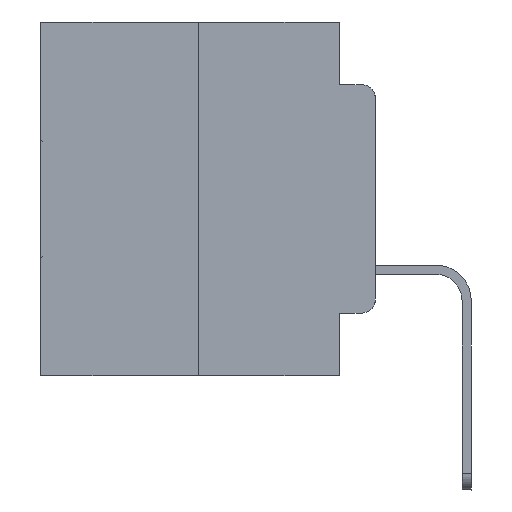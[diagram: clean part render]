
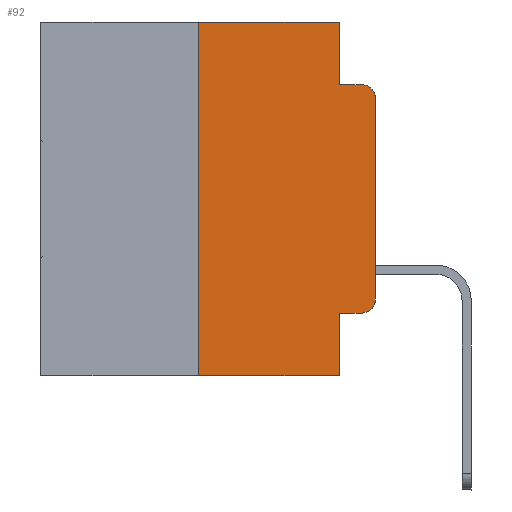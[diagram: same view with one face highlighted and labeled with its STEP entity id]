
A CAD part, left-side view. The second image highlights one B-rep face of the part: STEP entity #92.
In plain terms, the highlighted planar face has unit normal (-1, 0, 0).
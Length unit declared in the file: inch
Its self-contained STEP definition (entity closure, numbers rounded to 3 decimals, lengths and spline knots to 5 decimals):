
#92 = ADVANCED_FACE ( 'NONE', ( #2176 ), #473, .F. ) ;
#256 = EDGE_CURVE ( 'NONE', #11930, #10990, #23237, .T. ) ;
#473 = PLANE ( 'NONE',  #17647 ) ;
#1039 = CARTESIAN_POINT ( 'NONE',  ( 0., 0.051, -0.4115 ) ) ;
#1094 = EDGE_CURVE ( 'NONE', #29498, #14457, #22455, .T. ) ;
#1279 = VERTEX_POINT ( 'NONE', #23457 ) ;
#1362 = LINE ( 'NONE', #1039, #8848 ) ;
#1425 = EDGE_CURVE ( 'NONE', #28348, #14457, #18538, .T. ) ;
#1909 = EDGE_CURVE ( 'NONE', #5322, #10990, #22056, .T. ) ;
#2176 = FACE_OUTER_BOUND ( 'NONE', #20905, .T. ) ;
#3009 = CARTESIAN_POINT ( 'NONE',  ( 0., 0.25, -0.5 ) ) ;
#3118 = DIRECTION ( 'NONE',  ( 0., -1., 0. ) ) ;
#3403 = CARTESIAN_POINT ( 'NONE',  ( 0., 0.25, 0. ) ) ;
#3767 = VECTOR ( 'NONE', #28983, 39.37008 ) ;
#3899 = EDGE_CURVE ( 'NONE', #11930, #1279, #1362, .T. ) ;
#4281 = CIRCLE ( 'NONE', #28212, 0.02 ) ;
#4400 = DIRECTION ( 'NONE',  ( 0., -1., 0. ) ) ;
#5033 = VECTOR ( 'NONE', #6907, 39.37008 ) ;
#5210 = LINE ( 'NONE', #12337, #28712 ) ;
#5239 = DIRECTION ( 'NONE',  ( 0., 0., -1. ) ) ;
#5322 = VERTEX_POINT ( 'NONE', #3009 ) ;
#5488 = VERTEX_POINT ( 'NONE', #15306 ) ;
#6361 = ORIENTED_EDGE ( 'NONE', *, *, #20065, .F. ) ;
#6907 = DIRECTION ( 'NONE',  ( 0., 0., -1. ) ) ;
#8386 = CARTESIAN_POINT ( 'NONE',  ( 0., 0.051, -0.0885 ) ) ;
#8848 = VECTOR ( 'NONE', #3118, 39.37008 ) ;
#9566 = ORIENTED_EDGE ( 'NONE', *, *, #24116, .F. ) ;
#9853 = CARTESIAN_POINT ( 'NONE',  ( 0., 0.02, -0.0885 ) ) ;
#10698 = CARTESIAN_POINT ( 'NONE',  ( 0., 0.051, -0.4115 ) ) ;
#10990 = VERTEX_POINT ( 'NONE', #25135 ) ;
#11895 = ORIENTED_EDGE ( 'NONE', *, *, #3899, .T. ) ;
#11930 = VERTEX_POINT ( 'NONE', #10698 ) ;
#12065 = CARTESIAN_POINT ( 'NONE',  ( 0., 0., 0. ) ) ;
#12337 = CARTESIAN_POINT ( 'NONE',  ( 0., 0.051, 0. ) ) ;
#13448 = CARTESIAN_POINT ( 'NONE',  ( 0., 0.473, -0.5 ) ) ;
#13749 = LINE ( 'NONE', #25396, #27223 ) ;
#14352 = DIRECTION ( 'NONE',  ( 0., 0., 1. ) ) ;
#14457 = VERTEX_POINT ( 'NONE', #9853 ) ;
#14768 = EDGE_CURVE ( 'NONE', #15224, #20073, #18422, .T. ) ;
#14776 = ORIENTED_EDGE ( 'NONE', *, *, #17872, .T. ) ;
#14944 = ORIENTED_EDGE ( 'NONE', *, *, #1094, .F. ) ;
#15224 = VERTEX_POINT ( 'NONE', #3403 ) ;
#15306 = CARTESIAN_POINT ( 'NONE',  ( 0., 0., -0.3915 ) ) ;
#15640 = AXIS2_PLACEMENT_3D ( 'NONE', #19326, #21629, #17285 ) ;
#16142 = CARTESIAN_POINT ( 'NONE',  ( 0., 0.051, 0. ) ) ;
#16211 = DIRECTION ( 'NONE',  ( 0., 0., 1. ) ) ;
#16273 = DIRECTION ( 'NONE',  ( 1., 0., 0. ) ) ;
#16521 = CARTESIAN_POINT ( 'NONE',  ( 0., 0.051, 0. ) ) ;
#16740 = DIRECTION ( 'NONE',  ( -1., 0., 0. ) ) ;
#16800 = VECTOR ( 'NONE', #4400, 39.37008 ) ;
#17285 = DIRECTION ( 'NONE',  ( 0., 0., -1. ) ) ;
#17526 = LINE ( 'NONE', #12065, #25300 ) ;
#17647 = AXIS2_PLACEMENT_3D ( 'NONE', #18527, #16273, #5239 ) ;
#17810 = VECTOR ( 'NONE', #26818, 39.37008 ) ;
#17872 = EDGE_CURVE ( 'NONE', #1279, #5488, #4281, .T. ) ;
#17920 = EDGE_CURVE ( 'NONE', #5488, #28348, #17526, .T. ) ;
#18422 = LINE ( 'NONE', #24623, #3767 ) ;
#18527 = CARTESIAN_POINT ( 'NONE',  ( 0., 0.473, 0. ) ) ;
#18538 = CIRCLE ( 'NONE', #15640, 0.02 ) ;
#18884 = DIRECTION ( 'NONE',  ( 0., 0., -1. ) ) ;
#19151 = DIRECTION ( 'NONE',  ( 0., 0., -1. ) ) ;
#19326 = CARTESIAN_POINT ( 'NONE',  ( 0., 0.02, -0.1085 ) ) ;
#20065 = EDGE_CURVE ( 'NONE', #20073, #29498, #5210, .T. ) ;
#20073 = VERTEX_POINT ( 'NONE', #16521 ) ;
#20360 = CARTESIAN_POINT ( 'NONE',  ( 0., 0.051, -0.0885 ) ) ;
#20724 = ORIENTED_EDGE ( 'NONE', *, *, #1425, .T. ) ;
#20905 = EDGE_LOOP ( 'NONE', ( #24844, #20724, #14944, #6361, #22442, #9566, #27395, #25544, #11895, #14776 ) ) ;
#21629 = DIRECTION ( 'NONE',  ( -1., 0., 0. ) ) ;
#22056 = LINE ( 'NONE', #13448, #17810 ) ;
#22173 = CARTESIAN_POINT ( 'NONE',  ( 0., 0., -0.1085 ) ) ;
#22442 = ORIENTED_EDGE ( 'NONE', *, *, #14768, .F. ) ;
#22455 = LINE ( 'NONE', #20360, #16800 ) ;
#23237 = LINE ( 'NONE', #16142, #5033 ) ;
#23457 = CARTESIAN_POINT ( 'NONE',  ( 0., 0.02, -0.4115 ) ) ;
#24116 = EDGE_CURVE ( 'NONE', #5322, #15224, #13749, .T. ) ;
#24623 = CARTESIAN_POINT ( 'NONE',  ( 0., 0.473, 0. ) ) ;
#24844 = ORIENTED_EDGE ( 'NONE', *, *, #17920, .T. ) ;
#25135 = CARTESIAN_POINT ( 'NONE',  ( 0., 0.051, -0.5 ) ) ;
#25300 = VECTOR ( 'NONE', #14352, 39.37008 ) ;
#25396 = CARTESIAN_POINT ( 'NONE',  ( 0., 0.25, 0. ) ) ;
#25544 = ORIENTED_EDGE ( 'NONE', *, *, #256, .F. ) ;
#26818 = DIRECTION ( 'NONE',  ( 0., -1., 0. ) ) ;
#27223 = VECTOR ( 'NONE', #16211, 39.37008 ) ;
#27395 = ORIENTED_EDGE ( 'NONE', *, *, #1909, .T. ) ;
#27622 = CARTESIAN_POINT ( 'NONE',  ( 0., 0.02, -0.3915 ) ) ;
#28212 = AXIS2_PLACEMENT_3D ( 'NONE', #27622, #16740, #18884 ) ;
#28348 = VERTEX_POINT ( 'NONE', #22173 ) ;
#28712 = VECTOR ( 'NONE', #19151, 39.37008 ) ;
#28983 = DIRECTION ( 'NONE',  ( 0., -1., 0. ) ) ;
#29498 = VERTEX_POINT ( 'NONE', #8386 ) ;
